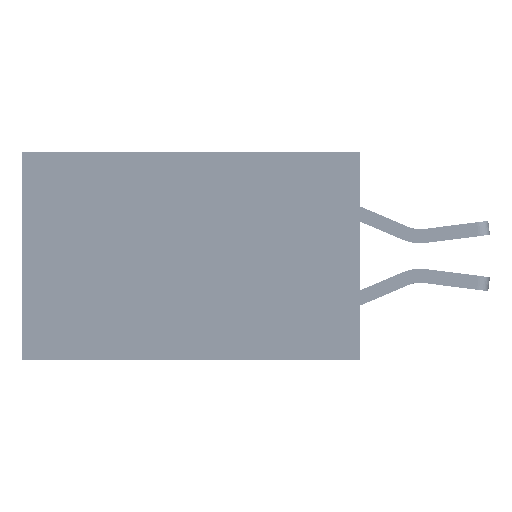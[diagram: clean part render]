
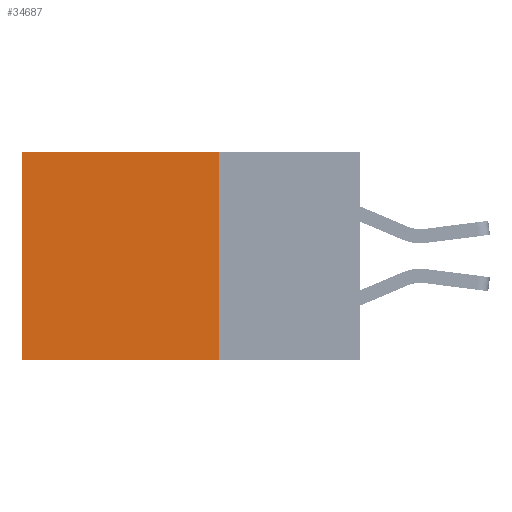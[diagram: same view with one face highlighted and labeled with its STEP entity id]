
A CAD part, left-side view. The second image highlights one B-rep face of the part: STEP entity #34687.
In plain terms, the highlighted planar face has unit normal (-1, 0, 0).
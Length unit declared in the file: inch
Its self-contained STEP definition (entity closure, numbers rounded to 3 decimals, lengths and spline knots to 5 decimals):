
#1064 = AXIS2_PLACEMENT_3D ( 'NONE', #10716, #34285, #22342 ) ;
#1885 = CARTESIAN_POINT ( 'NONE',  ( 0.2875, 0.6, 0. ) ) ;
#2816 = ORIENTED_EDGE ( 'NONE', *, *, #16233, .F. ) ;
#3186 = EDGE_CURVE ( 'NONE', #36718, #32225, #22999, .T. ) ;
#6630 = CARTESIAN_POINT ( 'NONE',  ( 0.2875, 0.25, 0. ) ) ;
#7296 = VECTOR ( 'NONE', #27863, 39.37008 ) ;
#9034 = EDGE_LOOP ( 'NONE', ( #21778, #17427, #2816, #14749 ) ) ;
#10716 = CARTESIAN_POINT ( 'NONE',  ( 0.2875, 0.25, 0. ) ) ;
#10923 = CARTESIAN_POINT ( 'NONE',  ( 0.2875, 0.6, -0.37 ) ) ;
#14264 = CARTESIAN_POINT ( 'NONE',  ( 0.2875, 0.25, 0. ) ) ;
#14749 = ORIENTED_EDGE ( 'NONE', *, *, #17755, .T. ) ;
#15717 = LINE ( 'NONE', #17712, #7296 ) ;
#15801 = EDGE_CURVE ( 'NONE', #20311, #32225, #19573, .T. ) ;
#16233 = EDGE_CURVE ( 'NONE', #34448, #20311, #15717, .T. ) ;
#17427 = ORIENTED_EDGE ( 'NONE', *, *, #15801, .F. ) ;
#17712 = CARTESIAN_POINT ( 'NONE',  ( 0.2875, 0.25, 0. ) ) ;
#17755 = EDGE_CURVE ( 'NONE', #34448, #36718, #19886, .T. ) ;
#19573 = LINE ( 'NONE', #36680, #28050 ) ;
#19789 = DIRECTION ( 'NONE',  ( 0., 1., 0. ) ) ;
#19886 = LINE ( 'NONE', #14264, #26091 ) ;
#20311 = VERTEX_POINT ( 'NONE', #38365 ) ;
#21778 = ORIENTED_EDGE ( 'NONE', *, *, #3186, .T. ) ;
#22342 = DIRECTION ( 'NONE',  ( 0., 0., -1. ) ) ;
#22999 = LINE ( 'NONE', #1885, #35206 ) ;
#24878 = DIRECTION ( 'NONE',  ( 0., 1., 0. ) ) ;
#25801 = PLANE ( 'NONE',  #1064 ) ;
#26091 = VECTOR ( 'NONE', #19789, 39.37008 ) ;
#27563 = FACE_OUTER_BOUND ( 'NONE', #9034, .T. ) ;
#27863 = DIRECTION ( 'NONE',  ( 0., 0., -1. ) ) ;
#28050 = VECTOR ( 'NONE', #24878, 39.37008 ) ;
#32225 = VERTEX_POINT ( 'NONE', #10923 ) ;
#32845 = CARTESIAN_POINT ( 'NONE',  ( 0.2875, 0.6, 0. ) ) ;
#34285 = DIRECTION ( 'NONE',  ( 1., 0., 0. ) ) ;
#34448 = VERTEX_POINT ( 'NONE', #6630 ) ;
#34687 = ADVANCED_FACE ( 'NONE', ( #27563 ), #25801, .F. ) ;
#35206 = VECTOR ( 'NONE', #37956, 39.37008 ) ;
#36680 = CARTESIAN_POINT ( 'NONE',  ( 0.2875, 0.25, -0.37 ) ) ;
#36718 = VERTEX_POINT ( 'NONE', #32845 ) ;
#37956 = DIRECTION ( 'NONE',  ( 0., 0., -1. ) ) ;
#38365 = CARTESIAN_POINT ( 'NONE',  ( 0.2875, 0.25, -0.37 ) ) ;
